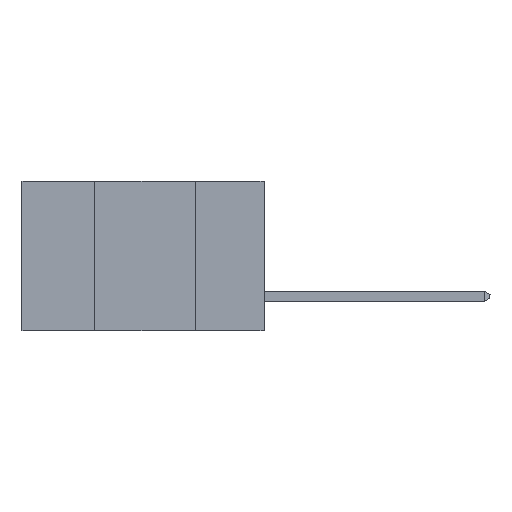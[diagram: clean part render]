
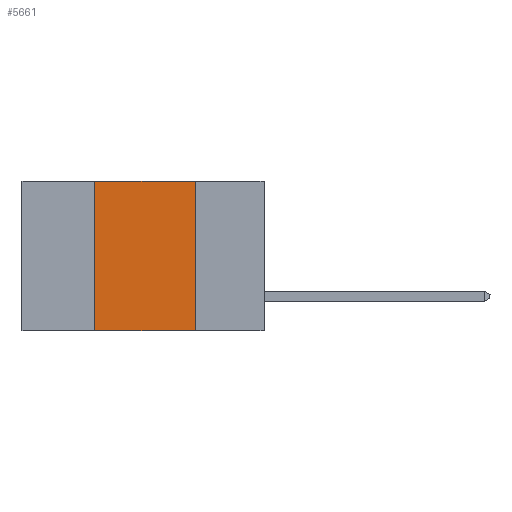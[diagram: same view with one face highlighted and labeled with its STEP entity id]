
A CAD part, left-side view. The second image highlights one B-rep face of the part: STEP entity #5661.
In plain terms, the highlighted planar face has unit normal (-1, 0, 0).
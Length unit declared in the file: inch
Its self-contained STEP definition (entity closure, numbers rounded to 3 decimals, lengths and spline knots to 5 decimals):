
#1940 = LINE ( 'NONE', #8766, #2826 ) ;
#2365 = ORIENTED_EDGE ( 'NONE', *, *, #5482, .F. ) ;
#2541 = AXIS2_PLACEMENT_3D ( 'NONE', #5623, #12614, #10556 ) ;
#2826 = VECTOR ( 'NONE', #8888, 39.37008 ) ;
#3014 = EDGE_LOOP ( 'NONE', ( #8519, #2365, #13010, #5331 ) ) ;
#3344 = EDGE_CURVE ( 'NONE', #6759, #4327, #6390, .T. ) ;
#3523 = CARTESIAN_POINT ( 'NONE',  ( 0., 0.42, 0. ) ) ;
#3851 = EDGE_CURVE ( 'NONE', #12127, #4327, #5447, .T. ) ;
#4327 = VERTEX_POINT ( 'NONE', #6676 ) ;
#4416 = VECTOR ( 'NONE', #7367, 39.37008 ) ;
#4428 = CARTESIAN_POINT ( 'NONE',  ( 0., 0.6, 0. ) ) ;
#4844 = EDGE_CURVE ( 'NONE', #6759, #12237, #1940, .T. ) ;
#5331 = ORIENTED_EDGE ( 'NONE', *, *, #3344, .T. ) ;
#5436 = VECTOR ( 'NONE', #9462, 39.37008 ) ;
#5447 = LINE ( 'NONE', #9267, #5436 ) ;
#5482 = EDGE_CURVE ( 'NONE', #12237, #12127, #8342, .T. ) ;
#5520 = CARTESIAN_POINT ( 'NONE',  ( 0., 0.6, -0.37 ) ) ;
#5623 = CARTESIAN_POINT ( 'NONE',  ( 0., 0.6, 0. ) ) ;
#5661 = ADVANCED_FACE ( 'NONE', ( #6549 ), #7747, .F. ) ;
#6324 = DIRECTION ( 'NONE',  ( 0., -1., 0. ) ) ;
#6390 = LINE ( 'NONE', #5520, #10411 ) ;
#6549 = FACE_OUTER_BOUND ( 'NONE', #3014, .T. ) ;
#6676 = CARTESIAN_POINT ( 'NONE',  ( 0., 0.17, -0.37 ) ) ;
#6759 = VERTEX_POINT ( 'NONE', #9484 ) ;
#7367 = DIRECTION ( 'NONE',  ( 0., -1., 0. ) ) ;
#7747 = PLANE ( 'NONE',  #2541 ) ;
#8342 = LINE ( 'NONE', #4428, #4416 ) ;
#8519 = ORIENTED_EDGE ( 'NONE', *, *, #3851, .F. ) ;
#8766 = CARTESIAN_POINT ( 'NONE',  ( 0., 0.42, -0.37 ) ) ;
#8888 = DIRECTION ( 'NONE',  ( 0., 0., 1. ) ) ;
#9267 = CARTESIAN_POINT ( 'NONE',  ( 0., 0.17, -0.37 ) ) ;
#9462 = DIRECTION ( 'NONE',  ( 0., 0., -1. ) ) ;
#9484 = CARTESIAN_POINT ( 'NONE',  ( 0., 0.42, -0.37 ) ) ;
#10411 = VECTOR ( 'NONE', #6324, 39.37008 ) ;
#10556 = DIRECTION ( 'NONE',  ( 0., 0., -1. ) ) ;
#11382 = CARTESIAN_POINT ( 'NONE',  ( 0., 0.17, 0. ) ) ;
#12127 = VERTEX_POINT ( 'NONE', #11382 ) ;
#12237 = VERTEX_POINT ( 'NONE', #3523 ) ;
#12614 = DIRECTION ( 'NONE',  ( 1., 0., 0. ) ) ;
#13010 = ORIENTED_EDGE ( 'NONE', *, *, #4844, .F. ) ;
